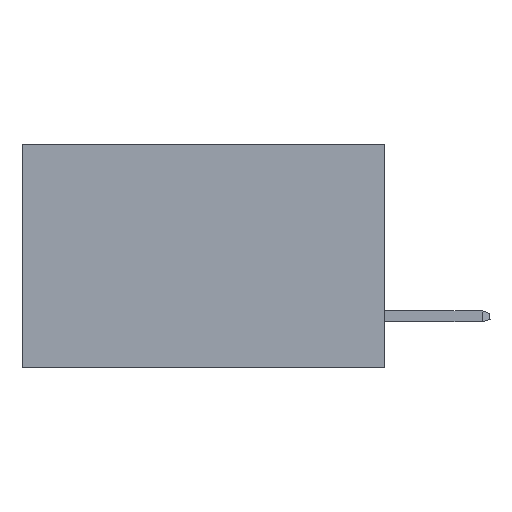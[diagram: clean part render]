
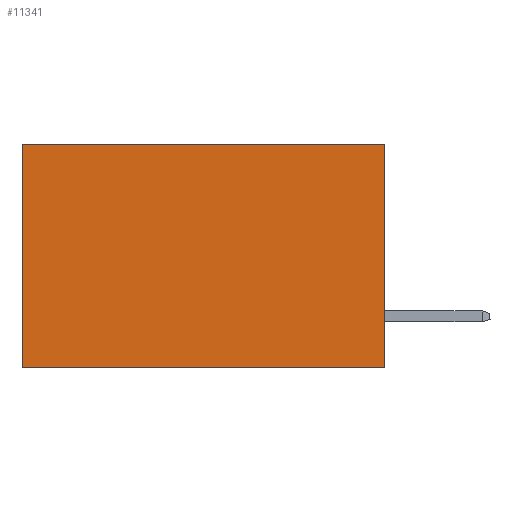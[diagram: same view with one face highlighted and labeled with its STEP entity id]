
A CAD part, left-side view. The second image highlights one B-rep face of the part: STEP entity #11341.
In plain terms, the highlighted planar face has unit normal (-1, 0, 0).
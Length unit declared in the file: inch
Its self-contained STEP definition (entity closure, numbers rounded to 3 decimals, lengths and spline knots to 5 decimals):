
#877 = CARTESIAN_POINT ( 'NONE',  ( 0.298, 0., -0.37 ) ) ;
#996 = DIRECTION ( 'NONE',  ( 0., 0., -1. ) ) ;
#1366 = CARTESIAN_POINT ( 'NONE',  ( 0.298, 0., 0. ) ) ;
#2402 = ORIENTED_EDGE ( 'NONE', *, *, #18412, .F. ) ;
#2869 = CARTESIAN_POINT ( 'NONE',  ( 0.298, 0.6, 0. ) ) ;
#2967 = CARTESIAN_POINT ( 'NONE',  ( 0.298, 0., -0.37 ) ) ;
#2991 = ORIENTED_EDGE ( 'NONE', *, *, #12191, .F. ) ;
#3496 = EDGE_CURVE ( 'NONE', #23992, #22103, #7079, .T. ) ;
#4234 = AXIS2_PLACEMENT_3D ( 'NONE', #1366, #25971, #15754 ) ;
#5393 = LINE ( 'NONE', #17436, #26019 ) ;
#7070 = CARTESIAN_POINT ( 'NONE',  ( 0.298, 0., 0. ) ) ;
#7079 = LINE ( 'NONE', #12532, #9342 ) ;
#7771 = EDGE_CURVE ( 'NONE', #22103, #22603, #25437, .T. ) ;
#9228 = CARTESIAN_POINT ( 'NONE',  ( 0.298, 0.6, 0. ) ) ;
#9342 = VECTOR ( 'NONE', #16648, 39.37008 ) ;
#9642 = LINE ( 'NONE', #2967, #24762 ) ;
#9768 = PLANE ( 'NONE',  #4234 ) ;
#11341 = ADVANCED_FACE ( 'NONE', ( #25065 ), #9768, .F. ) ;
#12191 = EDGE_CURVE ( 'NONE', #23992, #13710, #5393, .T. ) ;
#12532 = CARTESIAN_POINT ( 'NONE',  ( 0.298, 0., 0. ) ) ;
#13710 = VERTEX_POINT ( 'NONE', #877 ) ;
#15754 = DIRECTION ( 'NONE',  ( 0., 0., -1. ) ) ;
#16648 = DIRECTION ( 'NONE',  ( 0., 1., 0. ) ) ;
#16898 = EDGE_LOOP ( 'NONE', ( #24119, #2402, #2991, #24365 ) ) ;
#17436 = CARTESIAN_POINT ( 'NONE',  ( 0.298, 0., 0. ) ) ;
#18412 = EDGE_CURVE ( 'NONE', #13710, #22603, #9642, .T. ) ;
#19021 = VECTOR ( 'NONE', #996, 39.37008 ) ;
#20782 = CARTESIAN_POINT ( 'NONE',  ( 0.298, 0.6, -0.37 ) ) ;
#22103 = VERTEX_POINT ( 'NONE', #2869 ) ;
#22603 = VERTEX_POINT ( 'NONE', #20782 ) ;
#23566 = DIRECTION ( 'NONE',  ( 0., 1., 0. ) ) ;
#23992 = VERTEX_POINT ( 'NONE', #7070 ) ;
#24119 = ORIENTED_EDGE ( 'NONE', *, *, #7771, .T. ) ;
#24365 = ORIENTED_EDGE ( 'NONE', *, *, #3496, .T. ) ;
#24762 = VECTOR ( 'NONE', #23566, 39.37008 ) ;
#25065 = FACE_OUTER_BOUND ( 'NONE', #16898, .T. ) ;
#25437 = LINE ( 'NONE', #9228, #19021 ) ;
#25971 = DIRECTION ( 'NONE',  ( 1., 0., 0. ) ) ;
#26019 = VECTOR ( 'NONE', #26053, 39.37008 ) ;
#26053 = DIRECTION ( 'NONE',  ( 0., 0., -1. ) ) ;
